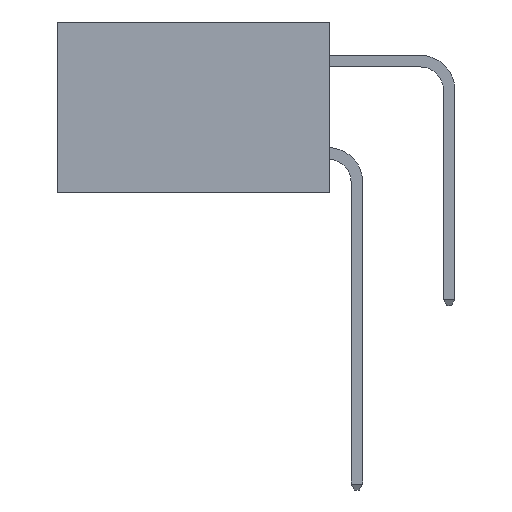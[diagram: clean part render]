
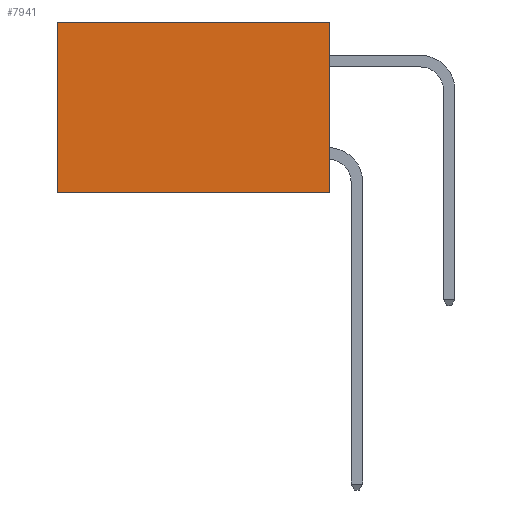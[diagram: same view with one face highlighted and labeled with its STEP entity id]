
A CAD part, left-side view. The second image highlights one B-rep face of the part: STEP entity #7941.
In plain terms, the highlighted planar face has unit normal (-1, 0, 0).
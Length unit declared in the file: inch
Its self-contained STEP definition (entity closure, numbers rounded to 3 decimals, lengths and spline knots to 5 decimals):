
#903 = CARTESIAN_POINT ( 'NONE',  ( 0.277, 0.59, -0.37 ) ) ;
#2106 = CARTESIAN_POINT ( 'NONE',  ( 0.277, 0., 0. ) ) ;
#2812 = CARTESIAN_POINT ( 'NONE',  ( 0.277, 0., -0.37 ) ) ;
#3685 = FACE_OUTER_BOUND ( 'NONE', #16603, .T. ) ;
#3969 = LINE ( 'NONE', #17314, #21572 ) ;
#4647 = ORIENTED_EDGE ( 'NONE', *, *, #17097, .F. ) ;
#4915 = EDGE_CURVE ( 'NONE', #16861, #13685, #3969, .T. ) ;
#5255 = LINE ( 'NONE', #2812, #18748 ) ;
#6707 = DIRECTION ( 'NONE',  ( 1., 0., 0. ) ) ;
#7050 = VECTOR ( 'NONE', #12861, 39.37008 ) ;
#7114 = CARTESIAN_POINT ( 'NONE',  ( 0.277, 0.59, -0.37 ) ) ;
#7941 = ADVANCED_FACE ( 'NONE', ( #3685 ), #22485, .F. ) ;
#8457 = VECTOR ( 'NONE', #21299, 39.37008 ) ;
#11895 = CARTESIAN_POINT ( 'NONE',  ( 0.277, 0., -0.37 ) ) ;
#11977 = AXIS2_PLACEMENT_3D ( 'NONE', #11895, #6707, #19066 ) ;
#12239 = CARTESIAN_POINT ( 'NONE',  ( 0.277, 0.59, 0. ) ) ;
#12861 = DIRECTION ( 'NONE',  ( 0., 0., -1. ) ) ;
#13069 = LINE ( 'NONE', #7114, #8457 ) ;
#13685 = VERTEX_POINT ( 'NONE', #12239 ) ;
#14864 = ORIENTED_EDGE ( 'NONE', *, *, #18621, .T. ) ;
#15083 = DIRECTION ( 'NONE',  ( 0., 1., 0. ) ) ;
#15881 = ORIENTED_EDGE ( 'NONE', *, *, #20627, .F. ) ;
#16462 = LINE ( 'NONE', #21712, #7050 ) ;
#16603 = EDGE_LOOP ( 'NONE', ( #14864, #4647, #15881, #21617 ) ) ;
#16861 = VERTEX_POINT ( 'NONE', #2106 ) ;
#17067 = VERTEX_POINT ( 'NONE', #903 ) ;
#17097 = EDGE_CURVE ( 'NONE', #17442, #17067, #5255, .T. ) ;
#17314 = CARTESIAN_POINT ( 'NONE',  ( 0.277, 0., 0. ) ) ;
#17442 = VERTEX_POINT ( 'NONE', #20072 ) ;
#17787 = DIRECTION ( 'NONE',  ( 0., 1., 0. ) ) ;
#18621 = EDGE_CURVE ( 'NONE', #13685, #17067, #13069, .T. ) ;
#18748 = VECTOR ( 'NONE', #15083, 39.37008 ) ;
#19066 = DIRECTION ( 'NONE',  ( 0., 0., -1. ) ) ;
#20072 = CARTESIAN_POINT ( 'NONE',  ( 0.277, 0., -0.37 ) ) ;
#20627 = EDGE_CURVE ( 'NONE', #16861, #17442, #16462, .T. ) ;
#21299 = DIRECTION ( 'NONE',  ( 0., 0., -1. ) ) ;
#21572 = VECTOR ( 'NONE', #17787, 39.37008 ) ;
#21617 = ORIENTED_EDGE ( 'NONE', *, *, #4915, .T. ) ;
#21712 = CARTESIAN_POINT ( 'NONE',  ( 0.277, 0., -0.37 ) ) ;
#22485 = PLANE ( 'NONE',  #11977 ) ;
